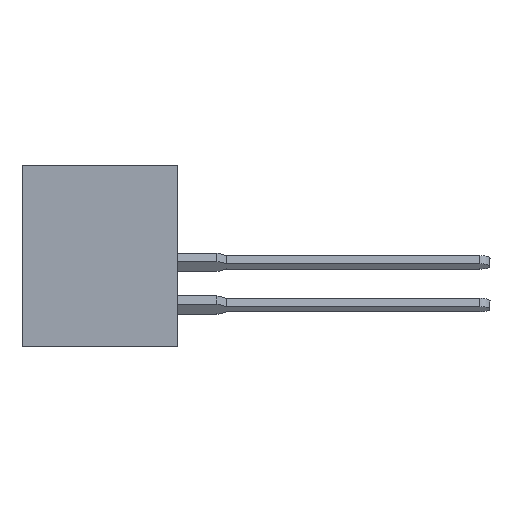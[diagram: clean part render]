
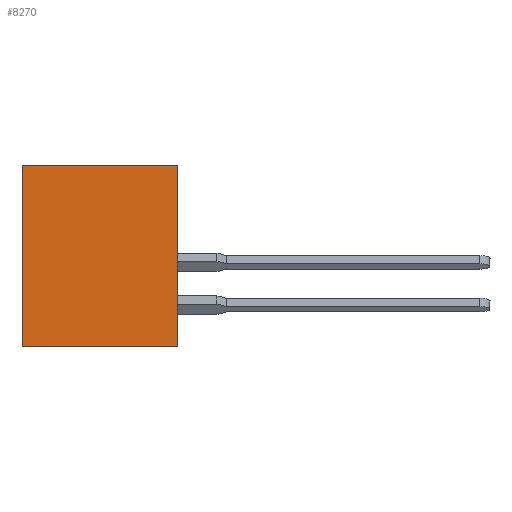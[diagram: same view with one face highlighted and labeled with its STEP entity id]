
A CAD part, left-side view. The second image highlights one B-rep face of the part: STEP entity #8270.
In plain terms, the highlighted planar face has unit normal (-1, 0, 0).
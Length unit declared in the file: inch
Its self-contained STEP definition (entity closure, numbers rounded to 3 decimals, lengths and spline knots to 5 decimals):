
#416 = DIRECTION ( 'NONE',  ( 0., -1., 0. ) ) ;
#898 = DIRECTION ( 'NONE',  ( 1., 0., 0. ) ) ;
#1096 = DIRECTION ( 'NONE',  ( 0., 0., -1. ) ) ;
#1272 = ORIENTED_EDGE ( 'NONE', *, *, #18638, .T. ) ;
#1915 = EDGE_CURVE ( 'NONE', #11079, #4912, #15302, .T. ) ;
#2311 = VERTEX_POINT ( 'NONE', #15466 ) ;
#3408 = ORIENTED_EDGE ( 'NONE', *, *, #14839, .F. ) ;
#3520 = CARTESIAN_POINT ( 'NONE',  ( 0., 0., 0. ) ) ;
#4212 = DIRECTION ( 'NONE',  ( 0., -1., 0. ) ) ;
#4792 = CARTESIAN_POINT ( 'NONE',  ( 0., 0.453, 0. ) ) ;
#4912 = VERTEX_POINT ( 'NONE', #3520 ) ;
#5403 = VECTOR ( 'NONE', #11186, 39.37008 ) ;
#6023 = FACE_OUTER_BOUND ( 'NONE', #16106, .T. ) ;
#6260 = ORIENTED_EDGE ( 'NONE', *, *, #1915, .T. ) ;
#7828 = VECTOR ( 'NONE', #4212, 39.37008 ) ;
#8270 = ADVANCED_FACE ( 'NONE', ( #6023 ), #10055, .F. ) ;
#8308 = VECTOR ( 'NONE', #12862, 39.37008 ) ;
#8544 = CARTESIAN_POINT ( 'NONE',  ( 0., 0.453, 0. ) ) ;
#9275 = ORIENTED_EDGE ( 'NONE', *, *, #14724, .F. ) ;
#10003 = CARTESIAN_POINT ( 'NONE',  ( 0., 0., 0. ) ) ;
#10036 = CARTESIAN_POINT ( 'NONE',  ( 0., 0., -0.531 ) ) ;
#10055 = PLANE ( 'NONE',  #16013 ) ;
#10067 = CARTESIAN_POINT ( 'NONE',  ( 0., 0.453, -0.531 ) ) ;
#10627 = VERTEX_POINT ( 'NONE', #19007 ) ;
#11079 = VERTEX_POINT ( 'NONE', #10036 ) ;
#11186 = DIRECTION ( 'NONE',  ( 0., 0., 1. ) ) ;
#11824 = LINE ( 'NONE', #10067, #7828 ) ;
#12862 = DIRECTION ( 'NONE',  ( 0., 0., 1. ) ) ;
#14724 = EDGE_CURVE ( 'NONE', #2311, #4912, #17664, .T. ) ;
#14839 = EDGE_CURVE ( 'NONE', #10627, #2311, #17795, .T. ) ;
#15302 = LINE ( 'NONE', #10003, #8308 ) ;
#15466 = CARTESIAN_POINT ( 'NONE',  ( 0., 0.453, 0. ) ) ;
#16013 = AXIS2_PLACEMENT_3D ( 'NONE', #8544, #898, #1096 ) ;
#16106 = EDGE_LOOP ( 'NONE', ( #6260, #9275, #3408, #1272 ) ) ;
#17073 = CARTESIAN_POINT ( 'NONE',  ( 0., 0.453, 0. ) ) ;
#17664 = LINE ( 'NONE', #4792, #18111 ) ;
#17795 = LINE ( 'NONE', #17073, #5403 ) ;
#18111 = VECTOR ( 'NONE', #416, 39.37008 ) ;
#18638 = EDGE_CURVE ( 'NONE', #10627, #11079, #11824, .T. ) ;
#19007 = CARTESIAN_POINT ( 'NONE',  ( 0., 0.453, -0.531 ) ) ;
